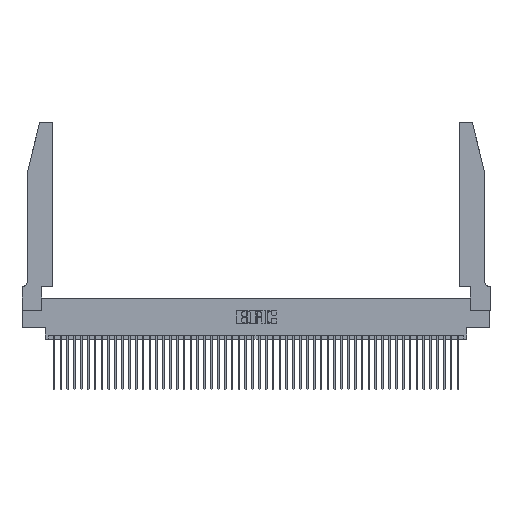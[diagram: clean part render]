
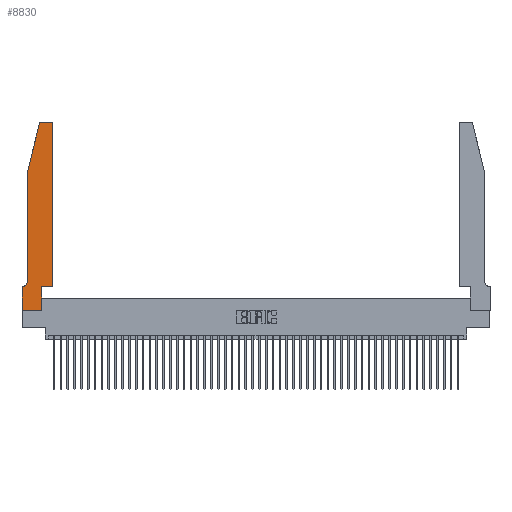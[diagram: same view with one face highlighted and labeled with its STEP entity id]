
A CAD part, top view. The second image highlights one B-rep face of the part: STEP entity #8830.
In plain terms, the highlighted planar face has unit normal (0, 0, 1).
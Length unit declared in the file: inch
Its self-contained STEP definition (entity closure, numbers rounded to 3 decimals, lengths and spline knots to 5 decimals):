
#337 = EDGE_LOOP ( 'NONE', ( #24621, #43641, #7181, #4145, #34826, #4774, #18752, #23000, #43173, #46752, #31368, #33798 ) ) ;
#522 = CIRCLE ( 'NONE', #39715, 0.03 ) ;
#1845 = EDGE_CURVE ( 'NONE', #16601, #34388, #522, .T. ) ;
#2313 = CARTESIAN_POINT ( 'NONE',  ( 0.2865, 0., 0.37 ) ) ;
#2761 = CIRCLE ( 'NONE', #10227, 0.07 ) ;
#2929 = CARTESIAN_POINT ( 'NONE',  ( 0.2605, 2.75, 0.37 ) ) ;
#3039 = VECTOR ( 'NONE', #40726, 39.37008 ) ;
#3087 = VERTEX_POINT ( 'NONE', #4076 ) ;
#3454 = VERTEX_POINT ( 'NONE', #29355 ) ;
#3886 = CARTESIAN_POINT ( 'NONE',  ( 0.2865, 0.35, 0.37 ) ) ;
#4072 = DIRECTION ( 'NONE',  ( 0., 0., 1. ) ) ;
#4076 = CARTESIAN_POINT ( 'NONE',  ( 0.25487, 2.72718, 0.37 ) ) ;
#4094 = EDGE_CURVE ( 'NONE', #14858, #5150, #42913, .T. ) ;
#4129 = DIRECTION ( 'NONE',  ( -0.239, -0.971, 0. ) ) ;
#4145 = ORIENTED_EDGE ( 'NONE', *, *, #4094, .T. ) ;
#4675 = VERTEX_POINT ( 'NONE', #16352 ) ;
#4774 = ORIENTED_EDGE ( 'NONE', *, *, #29633, .T. ) ;
#5150 = VERTEX_POINT ( 'NONE', #45730 ) ;
#6407 = FACE_OUTER_BOUND ( 'NONE', #337, .T. ) ;
#6835 = DIRECTION ( 'NONE',  ( -1., 0., 0. ) ) ;
#7181 = ORIENTED_EDGE ( 'NONE', *, *, #29834, .T. ) ;
#8830 = ADVANCED_FACE ( 'NONE', ( #6407 ), #43289, .T. ) ;
#8901 = EDGE_CURVE ( 'NONE', #5150, #42843, #2761, .T. ) ;
#9587 = CARTESIAN_POINT ( 'NONE',  ( 0.284, 2.75, 0.37 ) ) ;
#10227 = AXIS2_PLACEMENT_3D ( 'NONE', #36320, #13441, #40140 ) ;
#12046 = AXIS2_PLACEMENT_3D ( 'NONE', #27211, #4072, #31043 ) ;
#12287 = LINE ( 'NONE', #15681, #21356 ) ;
#13441 = DIRECTION ( 'NONE',  ( 0., 0., -1. ) ) ;
#14331 = EDGE_CURVE ( 'NONE', #41121, #3087, #20491, .T. ) ;
#14831 = VERTEX_POINT ( 'NONE', #41239 ) ;
#14858 = VERTEX_POINT ( 'NONE', #18618 ) ;
#15519 = EDGE_CURVE ( 'NONE', #15578, #14831, #41049, .T. ) ;
#15578 = VERTEX_POINT ( 'NONE', #41658 ) ;
#15681 = CARTESIAN_POINT ( 'NONE',  ( 0.0755, 2., 0.37 ) ) ;
#16352 = CARTESIAN_POINT ( 'NONE',  ( 0., 0., 0.37 ) ) ;
#16601 = VERTEX_POINT ( 'NONE', #38950 ) ;
#18208 = EDGE_CURVE ( 'NONE', #14831, #16601, #18774, .T. ) ;
#18558 = CARTESIAN_POINT ( 'NONE',  ( 0.4505, 0.35, 0.37 ) ) ;
#18618 = CARTESIAN_POINT ( 'NONE',  ( 0.0755, 2., 0.37 ) ) ;
#18752 = ORIENTED_EDGE ( 'NONE', *, *, #45815, .T. ) ;
#18774 = LINE ( 'NONE', #26206, #47897 ) ;
#19834 = CARTESIAN_POINT ( 'NONE',  ( 0.0055, 0.35, 0.37 ) ) ;
#20316 = CARTESIAN_POINT ( 'NONE',  ( 0.4205, 2.72, 0.37 ) ) ;
#20491 = CIRCLE ( 'NONE', #12046, 0.03 ) ;
#20561 = DIRECTION ( 'NONE',  ( 0., 0., 1. ) ) ;
#21356 = VECTOR ( 'NONE', #4129, 39.37008 ) ;
#21729 = EDGE_CURVE ( 'NONE', #4675, #34045, #33748, .T. ) ;
#22456 = CARTESIAN_POINT ( 'NONE',  ( 0.0755, 0.35, 0.37 ) ) ;
#22496 = EDGE_CURVE ( 'NONE', #34388, #41121, #29509, .T. ) ;
#23000 = ORIENTED_EDGE ( 'NONE', *, *, #21729, .T. ) ;
#24106 = CARTESIAN_POINT ( 'NONE',  ( 0.4205, 2.75, 0.37 ) ) ;
#24151 = DIRECTION ( 'NONE',  ( 1., 0., 0. ) ) ;
#24621 = ORIENTED_EDGE ( 'NONE', *, *, #22496, .T. ) ;
#24782 = CARTESIAN_POINT ( 'NONE',  ( 0.0755, 2., 0.37 ) ) ;
#25481 = CARTESIAN_POINT ( 'NONE',  ( 0., 0., 0.37 ) ) ;
#26206 = CARTESIAN_POINT ( 'NONE',  ( 0.4505, 0.35, 0.37 ) ) ;
#26281 = DIRECTION ( 'NONE',  ( -1., 0., 0. ) ) ;
#27211 = CARTESIAN_POINT ( 'NONE',  ( 0.284, 2.72, 0.37 ) ) ;
#28508 = EDGE_CURVE ( 'NONE', #34045, #15578, #49350, .T. ) ;
#28613 = DIRECTION ( 'NONE',  ( 0., -1., 0. ) ) ;
#29355 = CARTESIAN_POINT ( 'NONE',  ( 0., 0.35, 0.37 ) ) ;
#29509 = LINE ( 'NONE', #2929, #48432 ) ;
#29633 = EDGE_CURVE ( 'NONE', #42843, #3454, #40973, .T. ) ;
#29834 = EDGE_CURVE ( 'NONE', #3087, #14858, #12287, .T. ) ;
#30448 = VECTOR ( 'NONE', #30866, 39.37008 ) ;
#30866 = DIRECTION ( 'NONE',  ( 0., 1., 0. ) ) ;
#31043 = DIRECTION ( 'NONE',  ( 1., 0., 0. ) ) ;
#31368 = ORIENTED_EDGE ( 'NONE', *, *, #18208, .T. ) ;
#32873 = VECTOR ( 'NONE', #28613, 39.37008 ) ;
#33748 = LINE ( 'NONE', #25481, #3039 ) ;
#33798 = ORIENTED_EDGE ( 'NONE', *, *, #1845, .T. ) ;
#34045 = VERTEX_POINT ( 'NONE', #2313 ) ;
#34388 = VERTEX_POINT ( 'NONE', #24106 ) ;
#34545 = VECTOR ( 'NONE', #45175, 39.37008 ) ;
#34826 = ORIENTED_EDGE ( 'NONE', *, *, #8901, .T. ) ;
#36219 = VECTOR ( 'NONE', #49568, 39.37008 ) ;
#36320 = CARTESIAN_POINT ( 'NONE',  ( 0.0055, 0.42, 0.37 ) ) ;
#38950 = CARTESIAN_POINT ( 'NONE',  ( 0.4505, 2.72, 0.37 ) ) ;
#39488 = CARTESIAN_POINT ( 'NONE',  ( 0., 0.35, 0.37 ) ) ;
#39715 = AXIS2_PLACEMENT_3D ( 'NONE', #20316, #46866, #24151 ) ;
#39796 = VECTOR ( 'NONE', #26281, 39.37008 ) ;
#40140 = DIRECTION ( 'NONE',  ( -1., 0., 0. ) ) ;
#40726 = DIRECTION ( 'NONE',  ( 1., 0., 0. ) ) ;
#40973 = LINE ( 'NONE', #22456, #39796 ) ;
#41049 = LINE ( 'NONE', #18558, #34545 ) ;
#41121 = VERTEX_POINT ( 'NONE', #9587 ) ;
#41239 = CARTESIAN_POINT ( 'NONE',  ( 0.4505, 0.35, 0.37 ) ) ;
#41658 = CARTESIAN_POINT ( 'NONE',  ( 0.2865, 0.35, 0.37 ) ) ;
#42843 = VERTEX_POINT ( 'NONE', #19834 ) ;
#42913 = LINE ( 'NONE', #24782, #32873 ) ;
#43173 = ORIENTED_EDGE ( 'NONE', *, *, #28508, .T. ) ;
#43289 = PLANE ( 'NONE',  #44472 ) ;
#43641 = ORIENTED_EDGE ( 'NONE', *, *, #14331, .T. ) ;
#44472 = AXIS2_PLACEMENT_3D ( 'NONE', #39488, #20561, #47102 ) ;
#45175 = DIRECTION ( 'NONE',  ( 1., 0., 0. ) ) ;
#45257 = DIRECTION ( 'NONE',  ( 0., 1., 0. ) ) ;
#45730 = CARTESIAN_POINT ( 'NONE',  ( 0.0755, 0.42, 0.37 ) ) ;
#45781 = CARTESIAN_POINT ( 'NONE',  ( 0., 0., 0.37 ) ) ;
#45815 = EDGE_CURVE ( 'NONE', #3454, #4675, #46304, .T. ) ;
#46304 = LINE ( 'NONE', #45781, #36219 ) ;
#46752 = ORIENTED_EDGE ( 'NONE', *, *, #15519, .T. ) ;
#46866 = DIRECTION ( 'NONE',  ( 0., 0., 1. ) ) ;
#47102 = DIRECTION ( 'NONE',  ( 1., 0., 0. ) ) ;
#47897 = VECTOR ( 'NONE', #45257, 39.37008 ) ;
#48432 = VECTOR ( 'NONE', #6835, 39.37008 ) ;
#49350 = LINE ( 'NONE', #3886, #30448 ) ;
#49568 = DIRECTION ( 'NONE',  ( 0., -1., 0. ) ) ;
